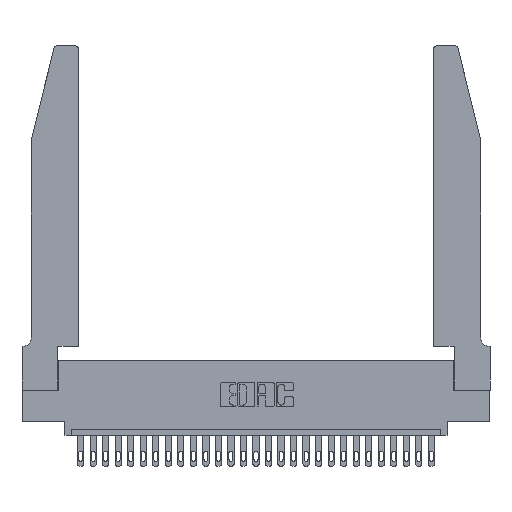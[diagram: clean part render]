
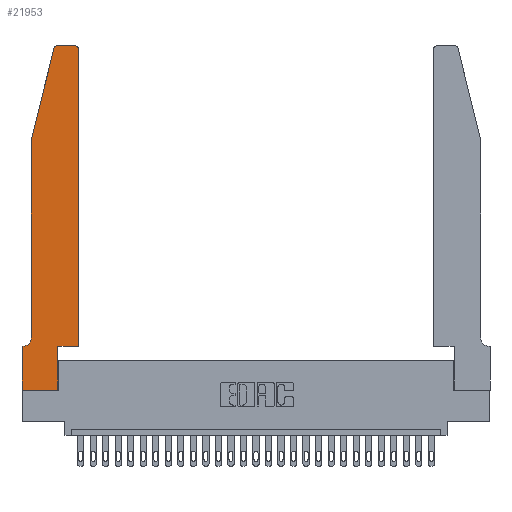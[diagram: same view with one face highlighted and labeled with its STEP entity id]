
A CAD part, top view. The second image highlights one B-rep face of the part: STEP entity #21953.
In plain terms, the highlighted planar face has unit normal (0, 0, 1).
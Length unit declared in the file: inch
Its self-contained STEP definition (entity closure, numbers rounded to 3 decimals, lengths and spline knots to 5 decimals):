
#1 = LINE ( 'NONE', #10020, #14703 ) ;
#399 = DIRECTION ( 'NONE',  ( 0., 1., 0. ) ) ;
#1268 = DIRECTION ( 'NONE',  ( 0., 0., 1. ) ) ;
#1432 = CARTESIAN_POINT ( 'NONE',  ( 0., 0., 0.37 ) ) ;
#1466 = CARTESIAN_POINT ( 'NONE',  ( 0.284, 2.72, 0.37 ) ) ;
#1519 = ORIENTED_EDGE ( 'NONE', *, *, #12330, .T. ) ;
#1821 = DIRECTION ( 'NONE',  ( 0., 1., 0. ) ) ;
#2005 = VECTOR ( 'NONE', #12547, 39.37008 ) ;
#2083 = EDGE_CURVE ( 'NONE', #15712, #7242, #14031, .T. ) ;
#2548 = DIRECTION ( 'NONE',  ( 0., -1., 0. ) ) ;
#2961 = CIRCLE ( 'NONE', #13178, 0.03 ) ;
#3401 = EDGE_CURVE ( 'NONE', #26075, #4611, #5773, .T. ) ;
#3831 = CARTESIAN_POINT ( 'NONE',  ( 0.0055, 0.35, 0.37 ) ) ;
#4611 = VERTEX_POINT ( 'NONE', #26719 ) ;
#5024 = CARTESIAN_POINT ( 'NONE',  ( 0.2865, 0.35, 0.37 ) ) ;
#5036 = CARTESIAN_POINT ( 'NONE',  ( 0., 0., 0.37 ) ) ;
#5044 = DIRECTION ( 'NONE',  ( 1., 0., 0. ) ) ;
#5123 = CARTESIAN_POINT ( 'NONE',  ( 0.2605, 2.75, 0.37 ) ) ;
#5773 = LINE ( 'NONE', #9901, #20122 ) ;
#5938 = ORIENTED_EDGE ( 'NONE', *, *, #24329, .T. ) ;
#6049 = VECTOR ( 'NONE', #7344, 39.37008 ) ;
#6147 = VECTOR ( 'NONE', #1821, 39.37008 ) ;
#6148 = AXIS2_PLACEMENT_3D ( 'NONE', #1466, #1268, #23326 ) ;
#6210 = ORIENTED_EDGE ( 'NONE', *, *, #2083, .T. ) ;
#6240 = ORIENTED_EDGE ( 'NONE', *, *, #24417, .T. ) ;
#6890 = ORIENTED_EDGE ( 'NONE', *, *, #21521, .T. ) ;
#7242 = VERTEX_POINT ( 'NONE', #19372 ) ;
#7344 = DIRECTION ( 'NONE',  ( -1., 0., 0. ) ) ;
#7912 = ORIENTED_EDGE ( 'NONE', *, *, #13980, .T. ) ;
#8390 = DIRECTION ( 'NONE',  ( 0., 0., 1. ) ) ;
#8962 = VECTOR ( 'NONE', #24931, 39.37008 ) ;
#9064 = PLANE ( 'NONE',  #26064 ) ;
#9246 = DIRECTION ( 'NONE',  ( 0., 0., 1. ) ) ;
#9582 = VERTEX_POINT ( 'NONE', #18156 ) ;
#9608 = VERTEX_POINT ( 'NONE', #13661 ) ;
#9836 = DIRECTION ( 'NONE',  ( 0., 0., -1. ) ) ;
#9839 = EDGE_CURVE ( 'NONE', #23087, #15712, #21696, .T. ) ;
#9901 = CARTESIAN_POINT ( 'NONE',  ( 0.0755, 0.35, 0.37 ) ) ;
#9953 = LINE ( 'NONE', #5036, #8962 ) ;
#10020 = CARTESIAN_POINT ( 'NONE',  ( 0.0755, 2., 0.37 ) ) ;
#10344 = EDGE_CURVE ( 'NONE', #12738, #23087, #9953, .T. ) ;
#10813 = CARTESIAN_POINT ( 'NONE',  ( 0.4505, 0.35, 0.37 ) ) ;
#11142 = ORIENTED_EDGE ( 'NONE', *, *, #9839, .T. ) ;
#11505 = ORIENTED_EDGE ( 'NONE', *, *, #22397, .T. ) ;
#11677 = CARTESIAN_POINT ( 'NONE',  ( 0.0755, 0.42, 0.37 ) ) ;
#12330 = EDGE_CURVE ( 'NONE', #23622, #16091, #1, .T. ) ;
#12547 = DIRECTION ( 'NONE',  ( 0., -1., 0. ) ) ;
#12738 = VERTEX_POINT ( 'NONE', #26792 ) ;
#12857 = CARTESIAN_POINT ( 'NONE',  ( 0.4205, 2.75, 0.37 ) ) ;
#13178 = AXIS2_PLACEMENT_3D ( 'NONE', #14978, #8390, #19083 ) ;
#13661 = CARTESIAN_POINT ( 'NONE',  ( 0.25487, 2.72718, 0.37 ) ) ;
#13733 = AXIS2_PLACEMENT_3D ( 'NONE', #22981, #9836, #23279 ) ;
#13980 = EDGE_CURVE ( 'NONE', #23996, #9582, #25208, .T. ) ;
#14012 = ORIENTED_EDGE ( 'NONE', *, *, #3401, .T. ) ;
#14031 = LINE ( 'NONE', #17620, #27080 ) ;
#14703 = VECTOR ( 'NONE', #2548, 39.37008 ) ;
#14978 = CARTESIAN_POINT ( 'NONE',  ( 0.4205, 2.72, 0.37 ) ) ;
#15242 = CARTESIAN_POINT ( 'NONE',  ( 0.2865, 0., 0.37 ) ) ;
#15700 = LINE ( 'NONE', #1432, #2005 ) ;
#15712 = VERTEX_POINT ( 'NONE', #5024 ) ;
#15858 = EDGE_CURVE ( 'NONE', #9582, #9608, #27862, .T. ) ;
#16091 = VERTEX_POINT ( 'NONE', #11677 ) ;
#16652 = CARTESIAN_POINT ( 'NONE',  ( 0.4505, 2.72, 0.37 ) ) ;
#17274 = DIRECTION ( 'NONE',  ( -0.239, -0.971, 0. ) ) ;
#17495 = FACE_OUTER_BOUND ( 'NONE', #27799, .T. ) ;
#17594 = VERTEX_POINT ( 'NONE', #16652 ) ;
#17620 = CARTESIAN_POINT ( 'NONE',  ( 0.4505, 0.35, 0.37 ) ) ;
#17748 = LINE ( 'NONE', #10813, #6147 ) ;
#18156 = CARTESIAN_POINT ( 'NONE',  ( 0.284, 2.75, 0.37 ) ) ;
#19083 = DIRECTION ( 'NONE',  ( 1., 0., 0. ) ) ;
#19266 = CARTESIAN_POINT ( 'NONE',  ( 0.0755, 2., 0.37 ) ) ;
#19372 = CARTESIAN_POINT ( 'NONE',  ( 0.4505, 0.35, 0.37 ) ) ;
#19383 = EDGE_CURVE ( 'NONE', #17594, #23996, #2961, .T. ) ;
#20104 = DIRECTION ( 'NONE',  ( -1., 0., 0. ) ) ;
#20122 = VECTOR ( 'NONE', #20104, 39.37008 ) ;
#20208 = ORIENTED_EDGE ( 'NONE', *, *, #15858, .T. ) ;
#20293 = CARTESIAN_POINT ( 'NONE',  ( 0.0755, 2., 0.37 ) ) ;
#21521 = EDGE_CURVE ( 'NONE', #16091, #26075, #27127, .T. ) ;
#21696 = LINE ( 'NONE', #28321, #25765 ) ;
#21953 = ADVANCED_FACE ( 'NONE', ( #17495 ), #9064, .T. ) ;
#21980 = LINE ( 'NONE', #19266, #25726 ) ;
#22158 = DIRECTION ( 'NONE',  ( 1., 0., 0. ) ) ;
#22397 = EDGE_CURVE ( 'NONE', #9608, #23622, #21980, .T. ) ;
#22981 = CARTESIAN_POINT ( 'NONE',  ( 0.0055, 0.42, 0.37 ) ) ;
#23087 = VERTEX_POINT ( 'NONE', #15242 ) ;
#23279 = DIRECTION ( 'NONE',  ( -1., 0., 0. ) ) ;
#23326 = DIRECTION ( 'NONE',  ( 1., 0., 0. ) ) ;
#23622 = VERTEX_POINT ( 'NONE', #20293 ) ;
#23996 = VERTEX_POINT ( 'NONE', #12857 ) ;
#24312 = CARTESIAN_POINT ( 'NONE',  ( 0., 0.35, 0.37 ) ) ;
#24329 = EDGE_CURVE ( 'NONE', #4611, #12738, #15700, .T. ) ;
#24417 = EDGE_CURVE ( 'NONE', #7242, #17594, #17748, .T. ) ;
#24931 = DIRECTION ( 'NONE',  ( 1., 0., 0. ) ) ;
#25208 = LINE ( 'NONE', #5123, #6049 ) ;
#25557 = ORIENTED_EDGE ( 'NONE', *, *, #10344, .T. ) ;
#25726 = VECTOR ( 'NONE', #17274, 39.37008 ) ;
#25765 = VECTOR ( 'NONE', #399, 39.37008 ) ;
#26064 = AXIS2_PLACEMENT_3D ( 'NONE', #24312, #9246, #5044 ) ;
#26075 = VERTEX_POINT ( 'NONE', #3831 ) ;
#26719 = CARTESIAN_POINT ( 'NONE',  ( 0., 0.35, 0.37 ) ) ;
#26792 = CARTESIAN_POINT ( 'NONE',  ( 0., 0., 0.37 ) ) ;
#27080 = VECTOR ( 'NONE', #22158, 39.37008 ) ;
#27127 = CIRCLE ( 'NONE', #13733, 0.07 ) ;
#27741 = ORIENTED_EDGE ( 'NONE', *, *, #19383, .T. ) ;
#27799 = EDGE_LOOP ( 'NONE', ( #7912, #20208, #11505, #1519, #6890, #14012, #5938, #25557, #11142, #6210, #6240, #27741 ) ) ;
#27862 = CIRCLE ( 'NONE', #6148, 0.03 ) ;
#28321 = CARTESIAN_POINT ( 'NONE',  ( 0.2865, 0.35, 0.37 ) ) ;
